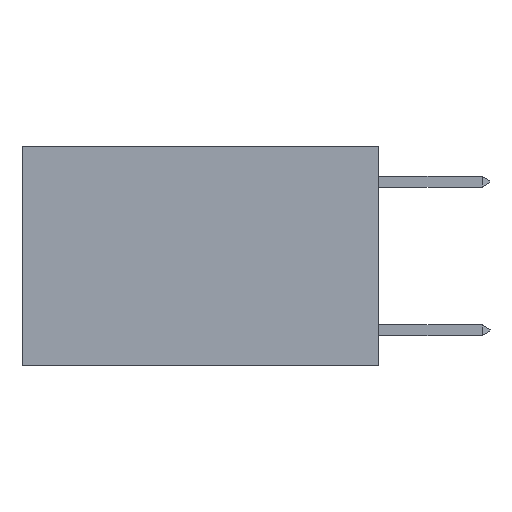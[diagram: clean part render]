
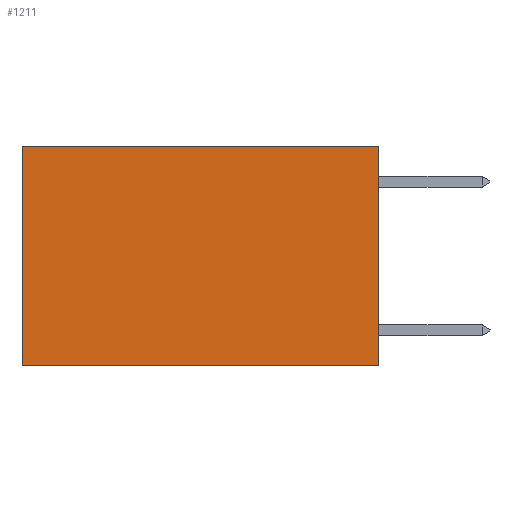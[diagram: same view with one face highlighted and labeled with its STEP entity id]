
A CAD part, left-side view. The second image highlights one B-rep face of the part: STEP entity #1211.
In plain terms, the highlighted planar face has unit normal (-1, 0, 0).
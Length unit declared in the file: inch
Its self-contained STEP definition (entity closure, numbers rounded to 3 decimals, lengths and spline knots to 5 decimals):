
#57 = DIRECTION ( 'NONE',  ( 1., 0., 0. ) ) ;
#60 = EDGE_CURVE ( 'NONE', #8188, #8812, #1197, .T. ) ;
#1197 = LINE ( 'NONE', #7668, #11303 ) ;
#1211 = ADVANCED_FACE ( 'NONE', ( #10970 ), #5100, .F. ) ;
#1260 = CARTESIAN_POINT ( 'NONE',  ( 0.2625, 0., 0. ) ) ;
#1997 = VECTOR ( 'NONE', #11990, 39.37008 ) ;
#2390 = DIRECTION ( 'NONE',  ( 0., 0., -1. ) ) ;
#2405 = CARTESIAN_POINT ( 'NONE',  ( 0.2625, 0., 0. ) ) ;
#2564 = CARTESIAN_POINT ( 'NONE',  ( 0.2625, 0.6, -0.37 ) ) ;
#2861 = CARTESIAN_POINT ( 'NONE',  ( 0.2625, 0., -0.37 ) ) ;
#3065 = ORIENTED_EDGE ( 'NONE', *, *, #11925, .T. ) ;
#3597 = EDGE_LOOP ( 'NONE', ( #3065, #9126, #6332, #5906 ) ) ;
#4029 = LINE ( 'NONE', #1260, #8822 ) ;
#4104 = CARTESIAN_POINT ( 'NONE',  ( 0.2625, 0., 0. ) ) ;
#4752 = DIRECTION ( 'NONE',  ( 0., 0., -1. ) ) ;
#4891 = EDGE_CURVE ( 'NONE', #10548, #10028, #8238, .T. ) ;
#5100 = PLANE ( 'NONE',  #8303 ) ;
#5906 = ORIENTED_EDGE ( 'NONE', *, *, #4891, .T. ) ;
#6332 = ORIENTED_EDGE ( 'NONE', *, *, #7813, .F. ) ;
#6475 = CARTESIAN_POINT ( 'NONE',  ( 0.2625, 0.6, 0. ) ) ;
#7592 = LINE ( 'NONE', #6475, #1997 ) ;
#7668 = CARTESIAN_POINT ( 'NONE',  ( 0.2625, 0., -0.37 ) ) ;
#7813 = EDGE_CURVE ( 'NONE', #10548, #8188, #4029, .T. ) ;
#7965 = VECTOR ( 'NONE', #11079, 39.37008 ) ;
#8188 = VERTEX_POINT ( 'NONE', #2861 ) ;
#8238 = LINE ( 'NONE', #2405, #7965 ) ;
#8303 = AXIS2_PLACEMENT_3D ( 'NONE', #4104, #57, #4752 ) ;
#8812 = VERTEX_POINT ( 'NONE', #2564 ) ;
#8822 = VECTOR ( 'NONE', #2390, 39.37008 ) ;
#9126 = ORIENTED_EDGE ( 'NONE', *, *, #60, .F. ) ;
#10028 = VERTEX_POINT ( 'NONE', #11748 ) ;
#10468 = CARTESIAN_POINT ( 'NONE',  ( 0.2625, 0., 0. ) ) ;
#10548 = VERTEX_POINT ( 'NONE', #10468 ) ;
#10970 = FACE_OUTER_BOUND ( 'NONE', #3597, .T. ) ;
#11079 = DIRECTION ( 'NONE',  ( 0., 1., 0. ) ) ;
#11303 = VECTOR ( 'NONE', #12676, 39.37008 ) ;
#11748 = CARTESIAN_POINT ( 'NONE',  ( 0.2625, 0.6, 0. ) ) ;
#11925 = EDGE_CURVE ( 'NONE', #10028, #8812, #7592, .T. ) ;
#11990 = DIRECTION ( 'NONE',  ( 0., 0., -1. ) ) ;
#12676 = DIRECTION ( 'NONE',  ( 0., 1., 0. ) ) ;
